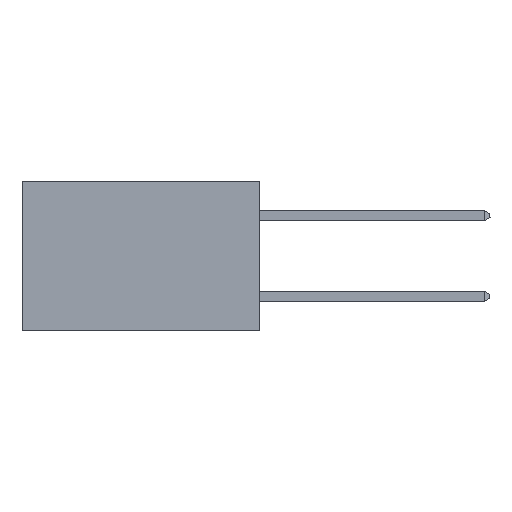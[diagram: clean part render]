
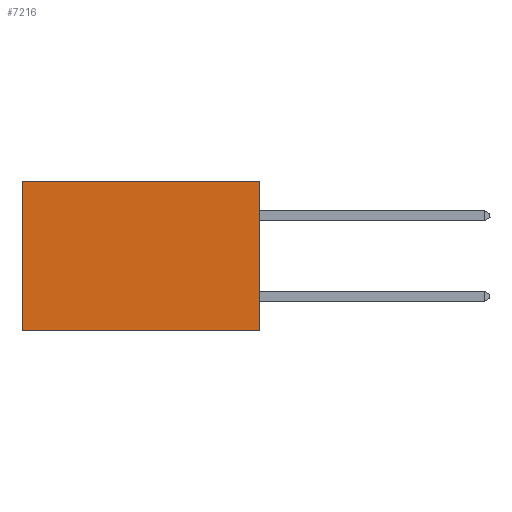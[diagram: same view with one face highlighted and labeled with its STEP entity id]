
A CAD part, left-side view. The second image highlights one B-rep face of the part: STEP entity #7216.
In plain terms, the highlighted planar face has unit normal (-1, 0, 0).
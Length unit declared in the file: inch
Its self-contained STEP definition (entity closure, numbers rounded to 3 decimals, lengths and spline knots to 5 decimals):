
#242 = CARTESIAN_POINT ( 'NONE',  ( 0.277, 0., -0.37 ) ) ;
#317 = VECTOR ( 'NONE', #21006, 39.37008 ) ;
#519 = LINE ( 'NONE', #16765, #28069 ) ;
#2976 = DIRECTION ( 'NONE',  ( 0., 0., -1. ) ) ;
#5812 = EDGE_CURVE ( 'NONE', #28020, #18359, #26529, .T. ) ;
#6083 = DIRECTION ( 'NONE',  ( 0., 0., -1. ) ) ;
#6942 = DIRECTION ( 'NONE',  ( 0., 1., 0. ) ) ;
#7161 = CARTESIAN_POINT ( 'NONE',  ( 0.277, 0., -0.37 ) ) ;
#7216 = ADVANCED_FACE ( 'NONE', ( #28092 ), #24198, .F. ) ;
#7277 = VECTOR ( 'NONE', #6083, 39.37008 ) ;
#8100 = ORIENTED_EDGE ( 'NONE', *, *, #5812, .F. ) ;
#8275 = ORIENTED_EDGE ( 'NONE', *, *, #11193, .T. ) ;
#9468 = CARTESIAN_POINT ( 'NONE',  ( 0.277, 0., 0. ) ) ;
#9471 = AXIS2_PLACEMENT_3D ( 'NONE', #242, #19031, #2976 ) ;
#10335 = CARTESIAN_POINT ( 'NONE',  ( 0.277, 0., 0. ) ) ;
#11124 = ORIENTED_EDGE ( 'NONE', *, *, #14743, .T. ) ;
#11193 = EDGE_CURVE ( 'NONE', #23528, #18359, #519, .T. ) ;
#11920 = EDGE_CURVE ( 'NONE', #13675, #28020, #27589, .T. ) ;
#13675 = VERTEX_POINT ( 'NONE', #9468 ) ;
#14532 = CARTESIAN_POINT ( 'NONE',  ( 0.277, 0.59, -0.37 ) ) ;
#14743 = EDGE_CURVE ( 'NONE', #13675, #23528, #33990, .T. ) ;
#16765 = CARTESIAN_POINT ( 'NONE',  ( 0.277, 0.59, -0.37 ) ) ;
#17736 = ORIENTED_EDGE ( 'NONE', *, *, #11920, .F. ) ;
#18359 = VERTEX_POINT ( 'NONE', #14532 ) ;
#19031 = DIRECTION ( 'NONE',  ( 1., 0., 0. ) ) ;
#21006 = DIRECTION ( 'NONE',  ( 0., 1., 0. ) ) ;
#21512 = CARTESIAN_POINT ( 'NONE',  ( 0.277, 0., -0.37 ) ) ;
#22032 = CARTESIAN_POINT ( 'NONE',  ( 0.277, 0., -0.37 ) ) ;
#23226 = CARTESIAN_POINT ( 'NONE',  ( 0.277, 0.59, 0. ) ) ;
#23528 = VERTEX_POINT ( 'NONE', #23226 ) ;
#24198 = PLANE ( 'NONE',  #9471 ) ;
#24636 = EDGE_LOOP ( 'NONE', ( #8275, #8100, #17736, #11124 ) ) ;
#26529 = LINE ( 'NONE', #7161, #32710 ) ;
#27589 = LINE ( 'NONE', #22032, #7277 ) ;
#28020 = VERTEX_POINT ( 'NONE', #21512 ) ;
#28069 = VECTOR ( 'NONE', #32561, 39.37008 ) ;
#28092 = FACE_OUTER_BOUND ( 'NONE', #24636, .T. ) ;
#32561 = DIRECTION ( 'NONE',  ( 0., 0., -1. ) ) ;
#32710 = VECTOR ( 'NONE', #6942, 39.37008 ) ;
#33990 = LINE ( 'NONE', #10335, #317 ) ;
